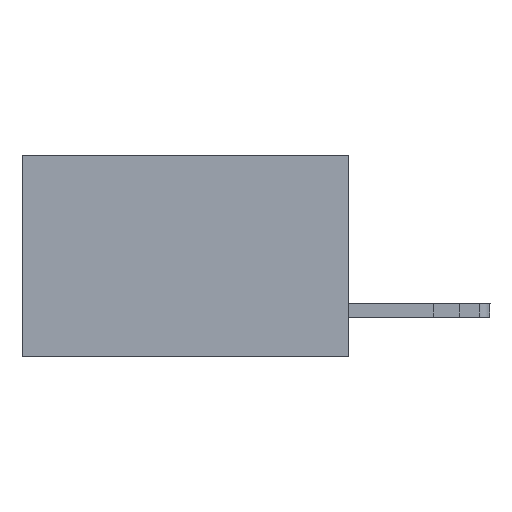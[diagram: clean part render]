
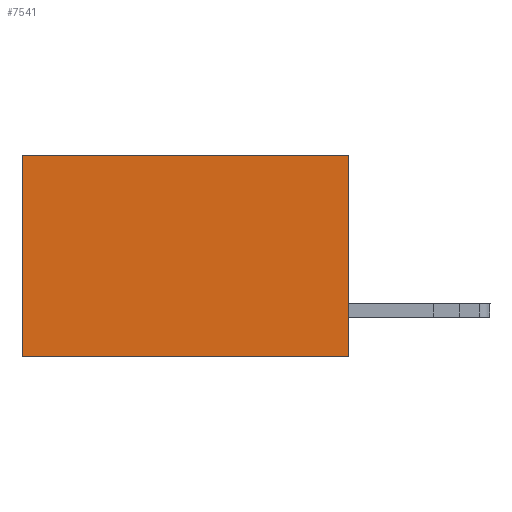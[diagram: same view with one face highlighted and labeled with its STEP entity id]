
A CAD part, left-side view. The second image highlights one B-rep face of the part: STEP entity #7541.
In plain terms, the highlighted planar face has unit normal (-1, 0, 0).
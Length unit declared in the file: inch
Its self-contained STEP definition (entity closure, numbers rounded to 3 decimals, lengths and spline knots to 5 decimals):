
#1055 = EDGE_CURVE ( 'NONE', #14398, #21535, #19762, .T. ) ;
#1596 = EDGE_CURVE ( 'NONE', #21535, #14459, #11095, .T. ) ;
#1901 = ORIENTED_EDGE ( 'NONE', *, *, #14647, .F. ) ;
#2938 = VECTOR ( 'NONE', #11616, 39.37008 ) ;
#3489 = ORIENTED_EDGE ( 'NONE', *, *, #1055, .T. ) ;
#3639 = ORIENTED_EDGE ( 'NONE', *, *, #9943, .F. ) ;
#5434 = EDGE_LOOP ( 'NONE', ( #14389, #1901, #3639, #3489 ) ) ;
#6846 = CARTESIAN_POINT ( 'NONE',  ( 0.298, 0., -0.37 ) ) ;
#7541 = ADVANCED_FACE ( 'NONE', ( #20344 ), #16286, .F. ) ;
#8011 = DIRECTION ( 'NONE',  ( 0., 1., 0. ) ) ;
#8674 = CARTESIAN_POINT ( 'NONE',  ( 0.298, 0.6, 0. ) ) ;
#8681 = VECTOR ( 'NONE', #16799, 39.37008 ) ;
#9871 = CARTESIAN_POINT ( 'NONE',  ( 0.298, 0., 0. ) ) ;
#9943 = EDGE_CURVE ( 'NONE', #14398, #13170, #16652, .T. ) ;
#11011 = CARTESIAN_POINT ( 'NONE',  ( 0.298, 0., 0. ) ) ;
#11095 = LINE ( 'NONE', #19697, #17289 ) ;
#11616 = DIRECTION ( 'NONE',  ( 0., 0., -1. ) ) ;
#11931 = VECTOR ( 'NONE', #8011, 39.37008 ) ;
#12581 = DIRECTION ( 'NONE',  ( 1., 0., 0. ) ) ;
#13170 = VERTEX_POINT ( 'NONE', #6846 ) ;
#14321 = LINE ( 'NONE', #21946, #8681 ) ;
#14389 = ORIENTED_EDGE ( 'NONE', *, *, #1596, .T. ) ;
#14390 = CARTESIAN_POINT ( 'NONE',  ( 0.298, 0., 0. ) ) ;
#14398 = VERTEX_POINT ( 'NONE', #14390 ) ;
#14459 = VERTEX_POINT ( 'NONE', #18033 ) ;
#14647 = EDGE_CURVE ( 'NONE', #13170, #14459, #14321, .T. ) ;
#15258 = AXIS2_PLACEMENT_3D ( 'NONE', #11011, #12581, #21486 ) ;
#16286 = PLANE ( 'NONE',  #15258 ) ;
#16652 = LINE ( 'NONE', #9871, #2938 ) ;
#16707 = CARTESIAN_POINT ( 'NONE',  ( 0.298, 0., 0. ) ) ;
#16799 = DIRECTION ( 'NONE',  ( 0., 1., 0. ) ) ;
#17289 = VECTOR ( 'NONE', #19839, 39.37008 ) ;
#18033 = CARTESIAN_POINT ( 'NONE',  ( 0.298, 0.6, -0.37 ) ) ;
#19697 = CARTESIAN_POINT ( 'NONE',  ( 0.298, 0.6, 0. ) ) ;
#19762 = LINE ( 'NONE', #16707, #11931 ) ;
#19839 = DIRECTION ( 'NONE',  ( 0., 0., -1. ) ) ;
#20344 = FACE_OUTER_BOUND ( 'NONE', #5434, .T. ) ;
#21486 = DIRECTION ( 'NONE',  ( 0., 0., -1. ) ) ;
#21535 = VERTEX_POINT ( 'NONE', #8674 ) ;
#21946 = CARTESIAN_POINT ( 'NONE',  ( 0.298, 0., -0.37 ) ) ;
